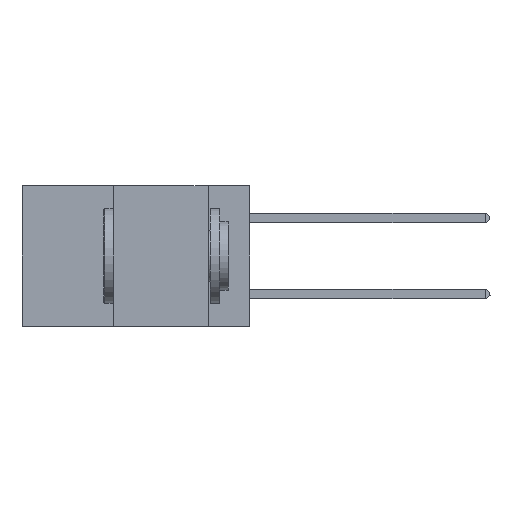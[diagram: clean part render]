
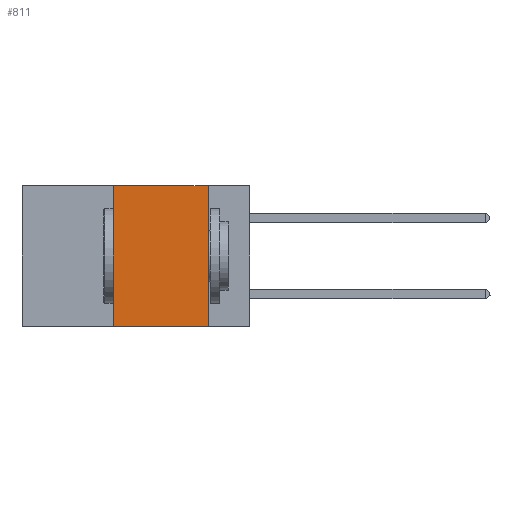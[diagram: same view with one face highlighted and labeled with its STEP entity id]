
A CAD part, left-side view. The second image highlights one B-rep face of the part: STEP entity #811.
In plain terms, the highlighted planar face has unit normal (-1, 0, 0).
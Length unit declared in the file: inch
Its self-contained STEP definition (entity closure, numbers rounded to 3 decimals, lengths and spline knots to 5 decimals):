
#672 = VERTEX_POINT ( 'NONE', #17330 ) ;
#686 = DIRECTION ( 'NONE',  ( 0., -1., 0. ) ) ;
#811 = ADVANCED_FACE ( 'NONE', ( #12694 ), #17162, .F. ) ;
#968 = ORIENTED_EDGE ( 'NONE', *, *, #18093, .F. ) ;
#1256 = DIRECTION ( 'NONE',  ( 0., 0., -1. ) ) ;
#1416 = EDGE_LOOP ( 'NONE', ( #12612, #968, #2344, #4148 ) ) ;
#1698 = LINE ( 'NONE', #9899, #6084 ) ;
#2344 = ORIENTED_EDGE ( 'NONE', *, *, #10814, .F. ) ;
#2557 = DIRECTION ( 'NONE',  ( 0., 0., 1. ) ) ;
#2638 = CARTESIAN_POINT ( 'NONE',  ( 0., 0.11, 0. ) ) ;
#2832 = DIRECTION ( 'NONE',  ( 0., 0., -1. ) ) ;
#2845 = LINE ( 'NONE', #14885, #8334 ) ;
#3336 = VECTOR ( 'NONE', #686, 39.37008 ) ;
#3348 = CARTESIAN_POINT ( 'NONE',  ( 0., 0.11, 0. ) ) ;
#4148 = ORIENTED_EDGE ( 'NONE', *, *, #9353, .T. ) ;
#5690 = CARTESIAN_POINT ( 'NONE',  ( 0., 0.6, 0. ) ) ;
#5722 = DIRECTION ( 'NONE',  ( 0., -1., 0. ) ) ;
#6084 = VECTOR ( 'NONE', #5722, 39.37008 ) ;
#6296 = CARTESIAN_POINT ( 'NONE',  ( 0., 0.6, -0.37 ) ) ;
#6565 = VERTEX_POINT ( 'NONE', #14816 ) ;
#8334 = VECTOR ( 'NONE', #2557, 39.37008 ) ;
#9353 = EDGE_CURVE ( 'NONE', #672, #11936, #17369, .T. ) ;
#9899 = CARTESIAN_POINT ( 'NONE',  ( 0., 0.6, 0. ) ) ;
#10575 = VERTEX_POINT ( 'NONE', #3348 ) ;
#10814 = EDGE_CURVE ( 'NONE', #672, #6565, #2845, .T. ) ;
#11209 = DIRECTION ( 'NONE',  ( 1., 0., 0. ) ) ;
#11228 = CARTESIAN_POINT ( 'NONE',  ( 0., 0.11, -0.37 ) ) ;
#11936 = VERTEX_POINT ( 'NONE', #11228 ) ;
#12141 = AXIS2_PLACEMENT_3D ( 'NONE', #5690, #11209, #2832 ) ;
#12612 = ORIENTED_EDGE ( 'NONE', *, *, #14648, .F. ) ;
#12694 = FACE_OUTER_BOUND ( 'NONE', #1416, .T. ) ;
#13667 = VECTOR ( 'NONE', #1256, 39.37008 ) ;
#14537 = LINE ( 'NONE', #2638, #13667 ) ;
#14648 = EDGE_CURVE ( 'NONE', #10575, #11936, #14537, .T. ) ;
#14816 = CARTESIAN_POINT ( 'NONE',  ( 0., 0.36, 0. ) ) ;
#14885 = CARTESIAN_POINT ( 'NONE',  ( 0., 0.36, 0. ) ) ;
#17162 = PLANE ( 'NONE',  #12141 ) ;
#17330 = CARTESIAN_POINT ( 'NONE',  ( 0., 0.36, -0.37 ) ) ;
#17369 = LINE ( 'NONE', #6296, #3336 ) ;
#18093 = EDGE_CURVE ( 'NONE', #6565, #10575, #1698, .T. ) ;
